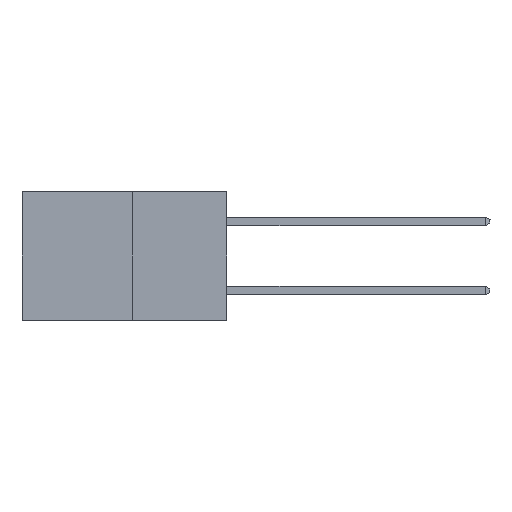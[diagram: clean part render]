
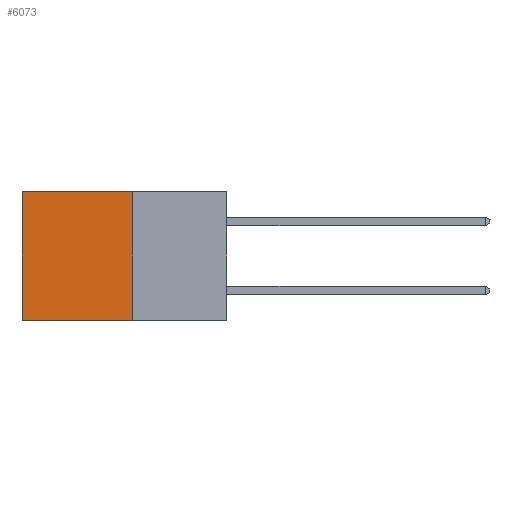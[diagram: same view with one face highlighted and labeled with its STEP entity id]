
A CAD part, left-side view. The second image highlights one B-rep face of the part: STEP entity #6073.
In plain terms, the highlighted planar face has unit normal (-1, 0, 0).
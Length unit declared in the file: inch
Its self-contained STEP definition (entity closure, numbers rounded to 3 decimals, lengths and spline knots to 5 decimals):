
#166 = ORIENTED_EDGE ( 'NONE', *, *, #339, .F. ) ;
#339 = EDGE_CURVE ( 'NONE', #7204, #1271, #6523, .T. ) ;
#371 = AXIS2_PLACEMENT_3D ( 'NONE', #3154, #6089, #1666 ) ;
#1082 = VERTEX_POINT ( 'NONE', #4767 ) ;
#1191 = CARTESIAN_POINT ( 'NONE',  ( 0.277, 0.27, 0. ) ) ;
#1233 = EDGE_LOOP ( 'NONE', ( #8700, #166, #8726, #3283 ) ) ;
#1271 = VERTEX_POINT ( 'NONE', #6754 ) ;
#1415 = VECTOR ( 'NONE', #6348, 39.37008 ) ;
#1666 = DIRECTION ( 'NONE',  ( 0., 0., -1. ) ) ;
#1992 = EDGE_CURVE ( 'NONE', #4040, #7204, #5101, .T. ) ;
#2045 = EDGE_CURVE ( 'NONE', #4040, #1082, #4179, .T. ) ;
#2633 = CARTESIAN_POINT ( 'NONE',  ( 0.277, 0.59, -0.37 ) ) ;
#2742 = VECTOR ( 'NONE', #8544, 39.37008 ) ;
#2860 = FACE_OUTER_BOUND ( 'NONE', #1233, .T. ) ;
#2897 = CARTESIAN_POINT ( 'NONE',  ( 0.277, 0.27, -0.37 ) ) ;
#3154 = CARTESIAN_POINT ( 'NONE',  ( 0.277, 0.27, -0.37 ) ) ;
#3283 = ORIENTED_EDGE ( 'NONE', *, *, #2045, .T. ) ;
#3560 = DIRECTION ( 'NONE',  ( 0., 1., 0. ) ) ;
#4040 = VERTEX_POINT ( 'NONE', #5785 ) ;
#4048 = CARTESIAN_POINT ( 'NONE',  ( 0.277, 0.27, -0.37 ) ) ;
#4179 = LINE ( 'NONE', #1191, #2742 ) ;
#4767 = CARTESIAN_POINT ( 'NONE',  ( 0.277, 0.59, 0. ) ) ;
#4943 = LINE ( 'NONE', #2633, #8041 ) ;
#5101 = LINE ( 'NONE', #6602, #1415 ) ;
#5327 = PLANE ( 'NONE',  #371 ) ;
#5785 = CARTESIAN_POINT ( 'NONE',  ( 0.277, 0.27, 0. ) ) ;
#6073 = ADVANCED_FACE ( 'NONE', ( #2860 ), #5327, .F. ) ;
#6089 = DIRECTION ( 'NONE',  ( 1., 0., 0. ) ) ;
#6348 = DIRECTION ( 'NONE',  ( 0., 0., -1. ) ) ;
#6523 = LINE ( 'NONE', #2897, #6723 ) ;
#6602 = CARTESIAN_POINT ( 'NONE',  ( 0.277, 0.27, -0.37 ) ) ;
#6723 = VECTOR ( 'NONE', #3560, 39.37008 ) ;
#6754 = CARTESIAN_POINT ( 'NONE',  ( 0.277, 0.59, -0.37 ) ) ;
#7204 = VERTEX_POINT ( 'NONE', #4048 ) ;
#8041 = VECTOR ( 'NONE', #8319, 39.37008 ) ;
#8319 = DIRECTION ( 'NONE',  ( 0., 0., -1. ) ) ;
#8544 = DIRECTION ( 'NONE',  ( 0., 1., 0. ) ) ;
#8700 = ORIENTED_EDGE ( 'NONE', *, *, #9103, .T. ) ;
#8726 = ORIENTED_EDGE ( 'NONE', *, *, #1992, .F. ) ;
#9103 = EDGE_CURVE ( 'NONE', #1082, #1271, #4943, .T. ) ;
